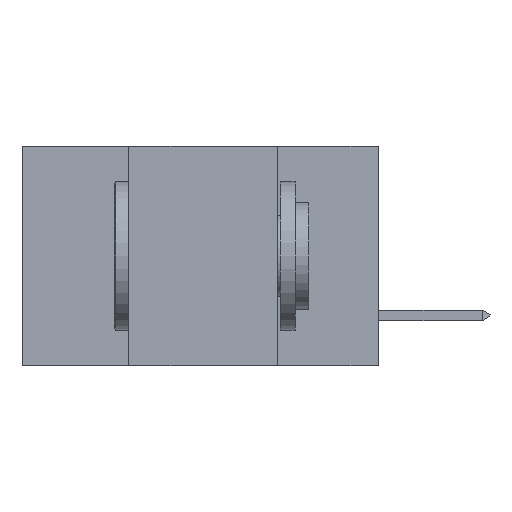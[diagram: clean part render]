
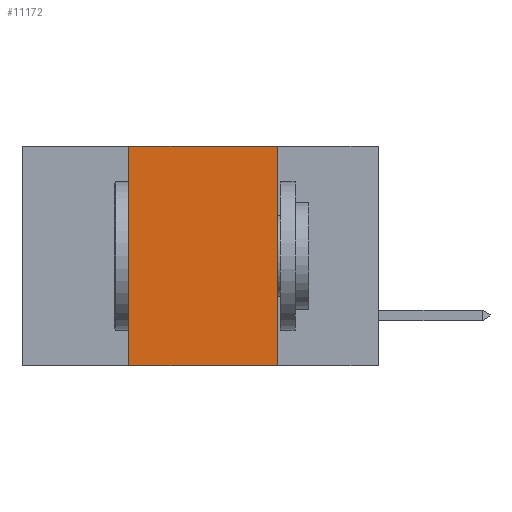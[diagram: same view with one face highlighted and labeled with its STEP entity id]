
A CAD part, left-side view. The second image highlights one B-rep face of the part: STEP entity #11172.
In plain terms, the highlighted planar face has unit normal (-1, 0, 0).
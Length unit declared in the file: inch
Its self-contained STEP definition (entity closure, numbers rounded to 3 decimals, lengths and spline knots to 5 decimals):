
#715 = EDGE_CURVE ( 'NONE', #23022, #1016, #16129, .T. ) ;
#1016 = VERTEX_POINT ( 'NONE', #14349 ) ;
#1359 = DIRECTION ( 'NONE',  ( 0., 0., 1. ) ) ;
#1555 = PLANE ( 'NONE',  #1790 ) ;
#1710 = CARTESIAN_POINT ( 'NONE',  ( 0., 0.17, 0. ) ) ;
#1790 = AXIS2_PLACEMENT_3D ( 'NONE', #18055, #16032, #20467 ) ;
#2759 = DIRECTION ( 'NONE',  ( 0., -1., 0. ) ) ;
#2793 = ORIENTED_EDGE ( 'NONE', *, *, #715, .F. ) ;
#2822 = EDGE_CURVE ( 'NONE', #10421, #23022, #19272, .T. ) ;
#3301 = VECTOR ( 'NONE', #8112, 39.37008 ) ;
#5385 = LINE ( 'NONE', #19759, #8642 ) ;
#8112 = DIRECTION ( 'NONE',  ( 0., 0., -1. ) ) ;
#8642 = VECTOR ( 'NONE', #1359, 39.37008 ) ;
#9134 = CARTESIAN_POINT ( 'NONE',  ( 0., 0.6, 0. ) ) ;
#9350 = EDGE_CURVE ( 'NONE', #25454, #10421, #5385, .T. ) ;
#10421 = VERTEX_POINT ( 'NONE', #18607 ) ;
#11172 = ADVANCED_FACE ( 'NONE', ( #20082 ), #1555, .F. ) ;
#11745 = EDGE_CURVE ( 'NONE', #25454, #1016, #24335, .T. ) ;
#12118 = CARTESIAN_POINT ( 'NONE',  ( 0., 0.6, -0.37 ) ) ;
#13724 = EDGE_LOOP ( 'NONE', ( #2793, #21255, #21925, #24663 ) ) ;
#14349 = CARTESIAN_POINT ( 'NONE',  ( 0., 0.17, -0.37 ) ) ;
#16032 = DIRECTION ( 'NONE',  ( 1., 0., 0. ) ) ;
#16129 = LINE ( 'NONE', #22079, #3301 ) ;
#18055 = CARTESIAN_POINT ( 'NONE',  ( 0., 0.6, 0. ) ) ;
#18151 = VECTOR ( 'NONE', #2759, 39.37008 ) ;
#18607 = CARTESIAN_POINT ( 'NONE',  ( 0., 0.42, 0. ) ) ;
#19272 = LINE ( 'NONE', #9134, #18151 ) ;
#19759 = CARTESIAN_POINT ( 'NONE',  ( 0., 0.42, -0.37 ) ) ;
#19809 = VECTOR ( 'NONE', #26525, 39.37008 ) ;
#20082 = FACE_OUTER_BOUND ( 'NONE', #13724, .T. ) ;
#20467 = DIRECTION ( 'NONE',  ( 0., 0., -1. ) ) ;
#21255 = ORIENTED_EDGE ( 'NONE', *, *, #2822, .F. ) ;
#21925 = ORIENTED_EDGE ( 'NONE', *, *, #9350, .F. ) ;
#22079 = CARTESIAN_POINT ( 'NONE',  ( 0., 0.17, -0.37 ) ) ;
#23022 = VERTEX_POINT ( 'NONE', #1710 ) ;
#24335 = LINE ( 'NONE', #12118, #19809 ) ;
#24663 = ORIENTED_EDGE ( 'NONE', *, *, #11745, .T. ) ;
#25096 = CARTESIAN_POINT ( 'NONE',  ( 0., 0.42, -0.37 ) ) ;
#25454 = VERTEX_POINT ( 'NONE', #25096 ) ;
#26525 = DIRECTION ( 'NONE',  ( 0., -1., 0. ) ) ;
